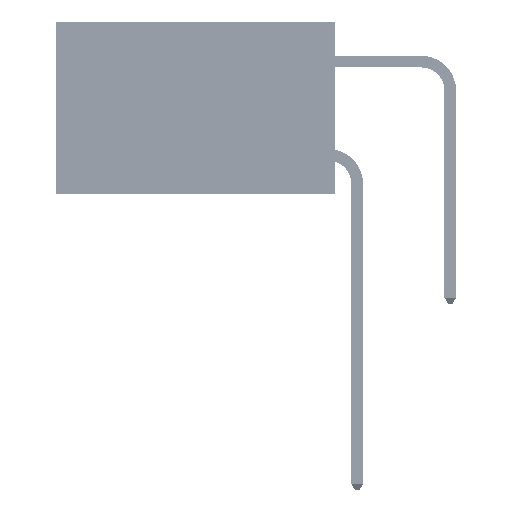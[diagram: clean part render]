
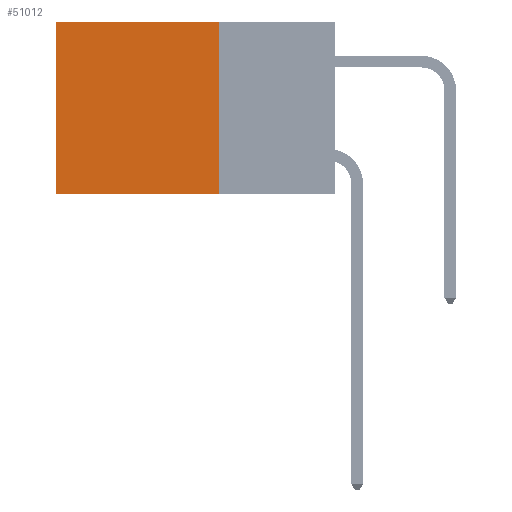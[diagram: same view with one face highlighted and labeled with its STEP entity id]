
A CAD part, left-side view. The second image highlights one B-rep face of the part: STEP entity #51012.
In plain terms, the highlighted planar face has unit normal (-1, 0, 0).
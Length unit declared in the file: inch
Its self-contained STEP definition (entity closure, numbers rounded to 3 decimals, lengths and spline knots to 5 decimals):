
#241 = DIRECTION ( 'NONE',  ( 1., 0., 0. ) ) ;
#949 = DIRECTION ( 'NONE',  ( 0., 1., 0. ) ) ;
#4031 = EDGE_CURVE ( 'NONE', #34072, #50082, #36073, .T. ) ;
#4761 = DIRECTION ( 'NONE',  ( 0., 0., -1. ) ) ;
#5020 = LINE ( 'NONE', #12220, #30064 ) ;
#5068 = EDGE_LOOP ( 'NONE', ( #18804, #47733, #7562, #8577 ) ) ;
#5702 = VERTEX_POINT ( 'NONE', #38677 ) ;
#6040 = VECTOR ( 'NONE', #26260, 39.37008 ) ;
#7562 = ORIENTED_EDGE ( 'NONE', *, *, #4031, .F. ) ;
#7870 = CARTESIAN_POINT ( 'NONE',  ( 0.2875, 0.25, 0. ) ) ;
#8577 = ORIENTED_EDGE ( 'NONE', *, *, #43111, .T. ) ;
#8722 = LINE ( 'NONE', #45973, #41876 ) ;
#12220 = CARTESIAN_POINT ( 'NONE',  ( 0.2875, 0.6, 0. ) ) ;
#14142 = VECTOR ( 'NONE', #46999, 39.37008 ) ;
#18249 = LINE ( 'NONE', #30797, #6040 ) ;
#18804 = ORIENTED_EDGE ( 'NONE', *, *, #47707, .T. ) ;
#20225 = DIRECTION ( 'NONE',  ( 0., 0., -1. ) ) ;
#23988 = EDGE_CURVE ( 'NONE', #50082, #43463, #18249, .T. ) ;
#24088 = CARTESIAN_POINT ( 'NONE',  ( 0.2875, 0.6, -0.37 ) ) ;
#24196 = AXIS2_PLACEMENT_3D ( 'NONE', #49235, #241, #20225 ) ;
#26260 = DIRECTION ( 'NONE',  ( 0., 1., 0. ) ) ;
#28218 = PLANE ( 'NONE',  #24196 ) ;
#28935 = CARTESIAN_POINT ( 'NONE',  ( 0.2875, 0.25, -0.37 ) ) ;
#30064 = VECTOR ( 'NONE', #4761, 39.37008 ) ;
#30797 = CARTESIAN_POINT ( 'NONE',  ( 0.2875, 0.25, -0.37 ) ) ;
#34072 = VERTEX_POINT ( 'NONE', #7870 ) ;
#35015 = CARTESIAN_POINT ( 'NONE',  ( 0.2875, 0.25, 0. ) ) ;
#36073 = LINE ( 'NONE', #35015, #14142 ) ;
#38677 = CARTESIAN_POINT ( 'NONE',  ( 0.2875, 0.6, 0. ) ) ;
#41528 = FACE_OUTER_BOUND ( 'NONE', #5068, .T. ) ;
#41876 = VECTOR ( 'NONE', #949, 39.37008 ) ;
#43111 = EDGE_CURVE ( 'NONE', #34072, #5702, #8722, .T. ) ;
#43463 = VERTEX_POINT ( 'NONE', #24088 ) ;
#45973 = CARTESIAN_POINT ( 'NONE',  ( 0.2875, 0.25, 0. ) ) ;
#46999 = DIRECTION ( 'NONE',  ( 0., 0., -1. ) ) ;
#47707 = EDGE_CURVE ( 'NONE', #5702, #43463, #5020, .T. ) ;
#47733 = ORIENTED_EDGE ( 'NONE', *, *, #23988, .F. ) ;
#49235 = CARTESIAN_POINT ( 'NONE',  ( 0.2875, 0.25, 0. ) ) ;
#50082 = VERTEX_POINT ( 'NONE', #28935 ) ;
#51012 = ADVANCED_FACE ( 'NONE', ( #41528 ), #28218, .F. ) ;
